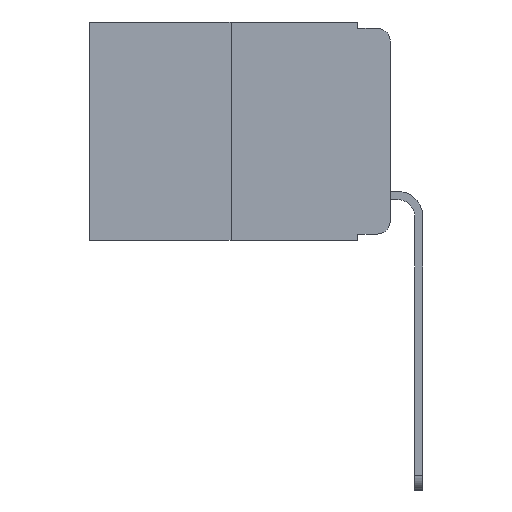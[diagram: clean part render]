
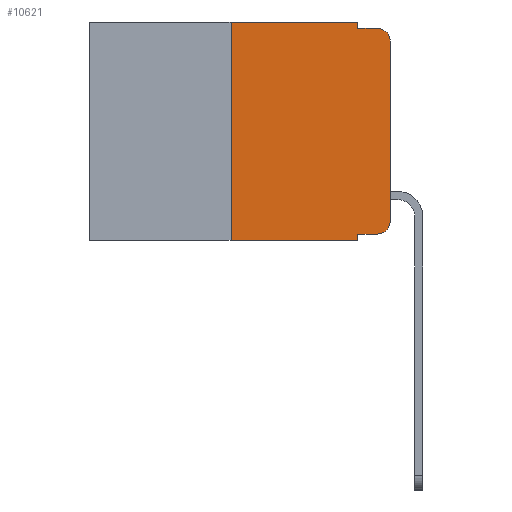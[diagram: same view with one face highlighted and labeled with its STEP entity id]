
A CAD part, left-side view. The second image highlights one B-rep face of the part: STEP entity #10621.
In plain terms, the highlighted planar face has unit normal (-1, 0, 0).
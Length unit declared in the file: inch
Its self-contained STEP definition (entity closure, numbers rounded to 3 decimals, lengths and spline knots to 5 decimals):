
#50 = VERTEX_POINT ( 'NONE', #1249 ) ;
#179 = VECTOR ( 'NONE', #780, 39.37008 ) ;
#423 = ORIENTED_EDGE ( 'NONE', *, *, #8518, .T. ) ;
#619 = LINE ( 'NONE', #3140, #8272 ) ;
#668 = DIRECTION ( 'NONE',  ( 0., 0., -1. ) ) ;
#671 = DIRECTION ( 'NONE',  ( 0., -1., 0. ) ) ;
#689 = CARTESIAN_POINT ( 'NONE',  ( 0., 0.051, 0. ) ) ;
#780 = DIRECTION ( 'NONE',  ( 0., 0., 1. ) ) ;
#1023 = ORIENTED_EDGE ( 'NONE', *, *, #3492, .T. ) ;
#1146 = VERTEX_POINT ( 'NONE', #8530 ) ;
#1249 = CARTESIAN_POINT ( 'NONE',  ( 0., 0.051, -0.343 ) ) ;
#1583 = CARTESIAN_POINT ( 'NONE',  ( 0., 0.02, -0.333 ) ) ;
#1925 = EDGE_CURVE ( 'NONE', #3092, #50, #12334, .T. ) ;
#1945 = ORIENTED_EDGE ( 'NONE', *, *, #10386, .T. ) ;
#1951 = CARTESIAN_POINT ( 'NONE',  ( 0., 0., -0.313 ) ) ;
#2010 = VERTEX_POINT ( 'NONE', #689 ) ;
#2094 = DIRECTION ( 'NONE',  ( 0., 0., 1. ) ) ;
#2524 = FACE_OUTER_BOUND ( 'NONE', #5530, .T. ) ;
#3062 = EDGE_CURVE ( 'NONE', #3092, #4496, #3644, .T. ) ;
#3092 = VERTEX_POINT ( 'NONE', #5526 ) ;
#3130 = LINE ( 'NONE', #8619, #179 ) ;
#3140 = CARTESIAN_POINT ( 'NONE',  ( 0., 0., 0. ) ) ;
#3292 = CARTESIAN_POINT ( 'NONE',  ( 0., 0.051, -0.01 ) ) ;
#3492 = EDGE_CURVE ( 'NONE', #4496, #11107, #8336, .T. ) ;
#3644 = LINE ( 'NONE', #9767, #8046 ) ;
#4164 = CIRCLE ( 'NONE', #11362, 0.02 ) ;
#4233 = EDGE_CURVE ( 'NONE', #12366, #1146, #3130, .T. ) ;
#4326 = CARTESIAN_POINT ( 'NONE',  ( 0., 0.02, -0.03 ) ) ;
#4378 = VECTOR ( 'NONE', #7149, 39.37008 ) ;
#4496 = VERTEX_POINT ( 'NONE', #1583 ) ;
#4729 = ORIENTED_EDGE ( 'NONE', *, *, #3062, .T. ) ;
#4755 = ORIENTED_EDGE ( 'NONE', *, *, #6792, .F. ) ;
#4997 = CARTESIAN_POINT ( 'NONE',  ( 0., 0.473, -0.343 ) ) ;
#5256 = DIRECTION ( 'NONE',  ( 0., -1., 0. ) ) ;
#5310 = DIRECTION ( 'NONE',  ( 0., 0., -1. ) ) ;
#5311 = DIRECTION ( 'NONE',  ( 1., 0., 0. ) ) ;
#5317 = DIRECTION ( 'NONE',  ( 0., 0., -1. ) ) ;
#5489 = VECTOR ( 'NONE', #668, 39.37008 ) ;
#5526 = CARTESIAN_POINT ( 'NONE',  ( 0., 0.051, -0.333 ) ) ;
#5530 = EDGE_LOOP ( 'NONE', ( #8249, #423, #7536, #6561, #4755, #9893, #1945, #7820, #4729, #1023 ) ) ;
#5609 = EDGE_CURVE ( 'NONE', #2010, #7514, #9798, .T. ) ;
#6077 = EDGE_CURVE ( 'NONE', #11107, #11886, #619, .T. ) ;
#6244 = CARTESIAN_POINT ( 'NONE',  ( 0., 0.473, 0. ) ) ;
#6561 = ORIENTED_EDGE ( 'NONE', *, *, #5609, .F. ) ;
#6601 = CARTESIAN_POINT ( 'NONE',  ( 0., 0.02, -0.313 ) ) ;
#6792 = EDGE_CURVE ( 'NONE', #1146, #2010, #9276, .T. ) ;
#7073 = CARTESIAN_POINT ( 'NONE',  ( 0., 0.02, -0.01 ) ) ;
#7127 = CARTESIAN_POINT ( 'NONE',  ( 0., 0.473, 0. ) ) ;
#7149 = DIRECTION ( 'NONE',  ( 0., -1., 0. ) ) ;
#7217 = LINE ( 'NONE', #4997, #9330 ) ;
#7369 = DIRECTION ( 'NONE',  ( -1., 0., 0. ) ) ;
#7514 = VERTEX_POINT ( 'NONE', #3292 ) ;
#7536 = ORIENTED_EDGE ( 'NONE', *, *, #9700, .F. ) ;
#7820 = ORIENTED_EDGE ( 'NONE', *, *, #1925, .F. ) ;
#8046 = VECTOR ( 'NONE', #5256, 39.37008 ) ;
#8084 = DIRECTION ( 'NONE',  ( 0., 0., -1. ) ) ;
#8249 = ORIENTED_EDGE ( 'NONE', *, *, #6077, .T. ) ;
#8272 = VECTOR ( 'NONE', #2094, 39.37008 ) ;
#8336 = CIRCLE ( 'NONE', #12195, 0.02 ) ;
#8481 = AXIS2_PLACEMENT_3D ( 'NONE', #7127, #5311, #11609 ) ;
#8518 = EDGE_CURVE ( 'NONE', #11886, #11309, #4164, .T. ) ;
#8530 = CARTESIAN_POINT ( 'NONE',  ( 0., 0.25, 0. ) ) ;
#8619 = CARTESIAN_POINT ( 'NONE',  ( 0., 0.25, 0. ) ) ;
#8973 = CARTESIAN_POINT ( 'NONE',  ( 0., 0., -0.03 ) ) ;
#9209 = VECTOR ( 'NONE', #671, 39.37008 ) ;
#9276 = LINE ( 'NONE', #6244, #4378 ) ;
#9319 = CARTESIAN_POINT ( 'NONE',  ( 0., 0.051, 0. ) ) ;
#9330 = VECTOR ( 'NONE', #12199, 39.37008 ) ;
#9477 = LINE ( 'NONE', #9488, #9209 ) ;
#9488 = CARTESIAN_POINT ( 'NONE',  ( 0., 0.051, -0.01 ) ) ;
#9700 = EDGE_CURVE ( 'NONE', #7514, #11309, #9477, .T. ) ;
#9767 = CARTESIAN_POINT ( 'NONE',  ( 0., 0.051, -0.333 ) ) ;
#9798 = LINE ( 'NONE', #10724, #12128 ) ;
#9893 = ORIENTED_EDGE ( 'NONE', *, *, #4233, .F. ) ;
#10270 = CARTESIAN_POINT ( 'NONE',  ( 0., 0.25, -0.343 ) ) ;
#10386 = EDGE_CURVE ( 'NONE', #12366, #50, #7217, .T. ) ;
#10621 = ADVANCED_FACE ( 'NONE', ( #2524 ), #10683, .F. ) ;
#10683 = PLANE ( 'NONE',  #8481 ) ;
#10716 = DIRECTION ( 'NONE',  ( -1., 0., 0. ) ) ;
#10724 = CARTESIAN_POINT ( 'NONE',  ( 0., 0.051, 0. ) ) ;
#11107 = VERTEX_POINT ( 'NONE', #1951 ) ;
#11309 = VERTEX_POINT ( 'NONE', #7073 ) ;
#11362 = AXIS2_PLACEMENT_3D ( 'NONE', #4326, #10716, #5310 ) ;
#11609 = DIRECTION ( 'NONE',  ( 0., 0., -1. ) ) ;
#11886 = VERTEX_POINT ( 'NONE', #8973 ) ;
#12128 = VECTOR ( 'NONE', #5317, 39.37008 ) ;
#12195 = AXIS2_PLACEMENT_3D ( 'NONE', #6601, #7369, #8084 ) ;
#12199 = DIRECTION ( 'NONE',  ( 0., -1., 0. ) ) ;
#12334 = LINE ( 'NONE', #9319, #5489 ) ;
#12366 = VERTEX_POINT ( 'NONE', #10270 ) ;
